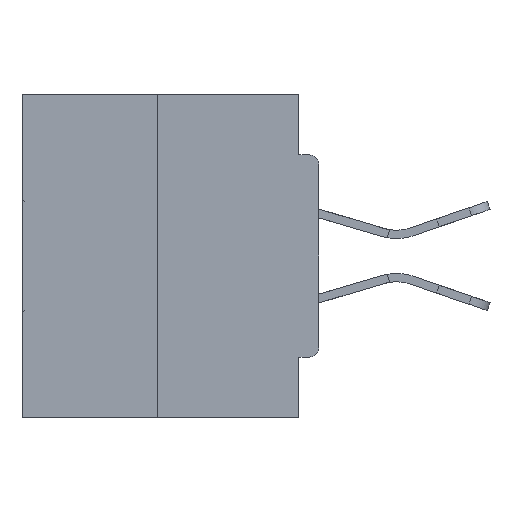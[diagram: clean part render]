
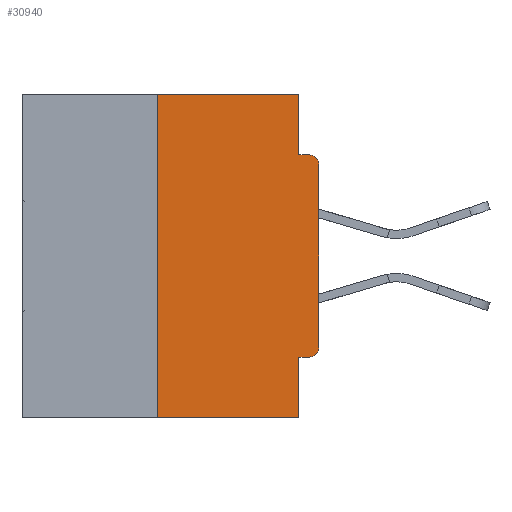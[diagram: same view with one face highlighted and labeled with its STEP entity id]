
A CAD part, left-side view. The second image highlights one B-rep face of the part: STEP entity #30940.
In plain terms, the highlighted planar face has unit normal (-1, 0, 0).
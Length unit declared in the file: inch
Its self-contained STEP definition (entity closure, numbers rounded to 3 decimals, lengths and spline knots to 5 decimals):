
#369 = CARTESIAN_POINT ( 'NONE',  ( 0., 0.25, -0.5 ) ) ;
#473 = PLANE ( 'NONE',  #32423 ) ;
#768 = DIRECTION ( 'NONE',  ( 0., 0., -1. ) ) ;
#1059 = DIRECTION ( 'NONE',  ( -1., 0., 0. ) ) ;
#1094 = EDGE_CURVE ( 'NONE', #2699, #36946, #4532, .T. ) ;
#1395 = EDGE_LOOP ( 'NONE', ( #18550, #15525, #9513, #14273, #33328, #13445, #28185, #4292, #20970, #30445 ) ) ;
#1511 = CARTESIAN_POINT ( 'NONE',  ( 0., 0., -0.4065 ) ) ;
#1749 = DIRECTION ( 'NONE',  ( -1., 0., 0. ) ) ;
#1843 = CARTESIAN_POINT ( 'NONE',  ( 0., 0.015, -0.4065 ) ) ;
#1881 = LINE ( 'NONE', #18061, #23587 ) ;
#2461 = VECTOR ( 'NONE', #27416, 39.37008 ) ;
#2699 = VERTEX_POINT ( 'NONE', #10880 ) ;
#3193 = CARTESIAN_POINT ( 'NONE',  ( 0., 0.25, 0. ) ) ;
#3271 = CARTESIAN_POINT ( 'NONE',  ( 0., 0.031, -0.5 ) ) ;
#3432 = CARTESIAN_POINT ( 'NONE',  ( 0., 0., -0.1085 ) ) ;
#3863 = LINE ( 'NONE', #3271, #10407 ) ;
#4292 = ORIENTED_EDGE ( 'NONE', *, *, #40777, .T. ) ;
#4532 = LINE ( 'NONE', #25807, #27204 ) ;
#4568 = DIRECTION ( 'NONE',  ( 0., -1., 0. ) ) ;
#4667 = EDGE_CURVE ( 'NONE', #22854, #6927, #27652, .T. ) ;
#4890 = EDGE_CURVE ( 'NONE', #8680, #33171, #6440, .T. ) ;
#5850 = EDGE_CURVE ( 'NONE', #38127, #8680, #28061, .T. ) ;
#6440 = LINE ( 'NONE', #30817, #39676 ) ;
#6633 = CARTESIAN_POINT ( 'NONE',  ( 0., 0.25, 0. ) ) ;
#6777 = EDGE_CURVE ( 'NONE', #34049, #2699, #26991, .T. ) ;
#6927 = VERTEX_POINT ( 'NONE', #3193 ) ;
#7095 = DIRECTION ( 'NONE',  ( 0., 0., -1. ) ) ;
#8195 = DIRECTION ( 'NONE',  ( 0., 0., -1. ) ) ;
#8680 = VERTEX_POINT ( 'NONE', #33801 ) ;
#9513 = ORIENTED_EDGE ( 'NONE', *, *, #33117, .T. ) ;
#10407 = VECTOR ( 'NONE', #19089, 39.37008 ) ;
#10880 = CARTESIAN_POINT ( 'NONE',  ( 0., 0., -0.3915 ) ) ;
#13191 = CARTESIAN_POINT ( 'NONE',  ( 0., 0.031, 0. ) ) ;
#13445 = ORIENTED_EDGE ( 'NONE', *, *, #6777, .T. ) ;
#14273 = ORIENTED_EDGE ( 'NONE', *, *, #20009, .F. ) ;
#15525 = ORIENTED_EDGE ( 'NONE', *, *, #4667, .F. ) ;
#16248 = DIRECTION ( 'NONE',  ( 0., 0., 1. ) ) ;
#17013 = DIRECTION ( 'NONE',  ( 1., 0., 0. ) ) ;
#17023 = VECTOR ( 'NONE', #20619, 39.37008 ) ;
#18061 = CARTESIAN_POINT ( 'NONE',  ( 0., 0.46, 0. ) ) ;
#18229 = CARTESIAN_POINT ( 'NONE',  ( 0., 0.015, -0.1085 ) ) ;
#18252 = EDGE_CURVE ( 'NONE', #34049, #38576, #24200, .T. ) ;
#18550 = ORIENTED_EDGE ( 'NONE', *, *, #24677, .F. ) ;
#19089 = DIRECTION ( 'NONE',  ( 0., 0., -1. ) ) ;
#19840 = CARTESIAN_POINT ( 'NONE',  ( 0., 0.031, 0. ) ) ;
#20009 = EDGE_CURVE ( 'NONE', #38576, #34162, #3863, .T. ) ;
#20122 = DIRECTION ( 'NONE',  ( 0., 0., -1. ) ) ;
#20619 = DIRECTION ( 'NONE',  ( 0., -1., 0. ) ) ;
#20970 = ORIENTED_EDGE ( 'NONE', *, *, #4890, .F. ) ;
#21159 = DIRECTION ( 'NONE',  ( 0., -1., 0. ) ) ;
#21578 = CARTESIAN_POINT ( 'NONE',  ( 0., 0.031, -0.5 ) ) ;
#22245 = FACE_OUTER_BOUND ( 'NONE', #1395, .T. ) ;
#22854 = VERTEX_POINT ( 'NONE', #369 ) ;
#23587 = VECTOR ( 'NONE', #21159, 39.37008 ) ;
#23937 = CIRCLE ( 'NONE', #24410, 0.015 ) ;
#24200 = LINE ( 'NONE', #1511, #2461 ) ;
#24410 = AXIS2_PLACEMENT_3D ( 'NONE', #18229, #1749, #8195 ) ;
#24677 = EDGE_CURVE ( 'NONE', #6927, #38127, #1881, .T. ) ;
#25422 = CARTESIAN_POINT ( 'NONE',  ( 0., 0.031, -0.4065 ) ) ;
#25807 = CARTESIAN_POINT ( 'NONE',  ( 0., 0., 0. ) ) ;
#26251 = DIRECTION ( 'NONE',  ( 0., 0., 1. ) ) ;
#26271 = CARTESIAN_POINT ( 'NONE',  ( 0., 0.46, 0. ) ) ;
#26870 = AXIS2_PLACEMENT_3D ( 'NONE', #33067, #1059, #7095 ) ;
#26991 = CIRCLE ( 'NONE', #26870, 0.015 ) ;
#27204 = VECTOR ( 'NONE', #16248, 39.37008 ) ;
#27416 = DIRECTION ( 'NONE',  ( 0., 1., 0. ) ) ;
#27652 = LINE ( 'NONE', #6633, #37625 ) ;
#28061 = LINE ( 'NONE', #19840, #39054 ) ;
#28185 = ORIENTED_EDGE ( 'NONE', *, *, #1094, .T. ) ;
#30445 = ORIENTED_EDGE ( 'NONE', *, *, #5850, .F. ) ;
#30817 = CARTESIAN_POINT ( 'NONE',  ( 0., 0., -0.0935 ) ) ;
#30922 = CARTESIAN_POINT ( 'NONE',  ( 0., 0.015, -0.0935 ) ) ;
#30940 = ADVANCED_FACE ( 'NONE', ( #22245 ), #473, .F. ) ;
#32423 = AXIS2_PLACEMENT_3D ( 'NONE', #26271, #17013, #20122 ) ;
#33067 = CARTESIAN_POINT ( 'NONE',  ( 0., 0.015, -0.3915 ) ) ;
#33117 = EDGE_CURVE ( 'NONE', #22854, #34162, #36540, .T. ) ;
#33171 = VERTEX_POINT ( 'NONE', #30922 ) ;
#33328 = ORIENTED_EDGE ( 'NONE', *, *, #18252, .F. ) ;
#33801 = CARTESIAN_POINT ( 'NONE',  ( 0., 0.031, -0.0935 ) ) ;
#34049 = VERTEX_POINT ( 'NONE', #1843 ) ;
#34162 = VERTEX_POINT ( 'NONE', #21578 ) ;
#36540 = LINE ( 'NONE', #39359, #17023 ) ;
#36946 = VERTEX_POINT ( 'NONE', #3432 ) ;
#37625 = VECTOR ( 'NONE', #26251, 39.37008 ) ;
#38127 = VERTEX_POINT ( 'NONE', #13191 ) ;
#38576 = VERTEX_POINT ( 'NONE', #25422 ) ;
#39054 = VECTOR ( 'NONE', #768, 39.37008 ) ;
#39359 = CARTESIAN_POINT ( 'NONE',  ( 0., 0.46, -0.5 ) ) ;
#39676 = VECTOR ( 'NONE', #4568, 39.37008 ) ;
#40777 = EDGE_CURVE ( 'NONE', #36946, #33171, #23937, .T. ) ;
